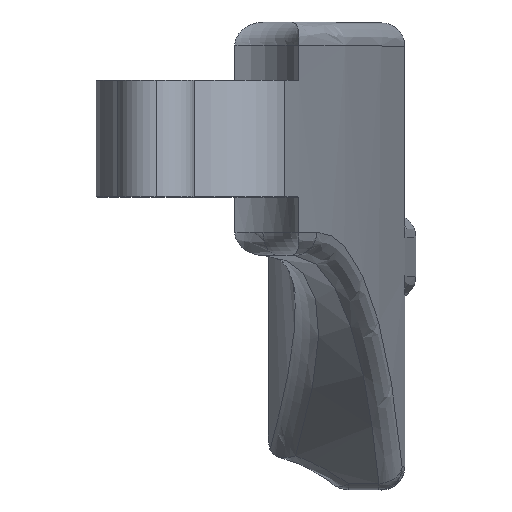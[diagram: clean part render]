
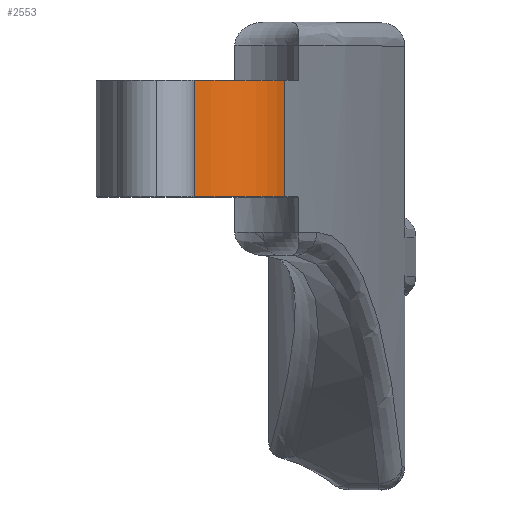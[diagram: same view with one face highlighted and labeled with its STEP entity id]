
A CAD part, top view. The second image highlights one B-rep face of the part: STEP entity #2553.
In plain terms, the highlighted cylindrical face has radius 12.6 mm (diameter 25.2 mm), a partial arc.
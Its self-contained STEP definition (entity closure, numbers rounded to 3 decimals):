
#46 = EDGE_LOOP ( 'NONE', ( #496, #1217, #1974, #1426 ) ) ;
#118 = EDGE_CURVE ( 'NONE', #2184, #1046, #1767, .T. ) ;
#164 = EDGE_CURVE ( 'NONE', #1065, #2184, #1087, .T. ) ;
#210 = LINE ( 'NONE', #1820, #586 ) ;
#295 = CIRCLE ( 'NONE', #1758, 12.6 ) ;
#458 = DIRECTION ( 'NONE',  ( 0., 1., 0. ) ) ;
#496 = ORIENTED_EDGE ( 'NONE', *, *, #118, .T. ) ;
#586 = VECTOR ( 'NONE', #1199, 1000. ) ;
#598 = FACE_OUTER_BOUND ( 'NONE', #46, .T. ) ;
#826 = CARTESIAN_POINT ( 'NONE',  ( 0., -60., 110. ) ) ;
#856 = DIRECTION ( 'NONE',  ( 0., -1., 0. ) ) ;
#911 = EDGE_CURVE ( 'NONE', #1065, #1109, #295, .T. ) ;
#976 = AXIS2_PLACEMENT_3D ( 'NONE', #1062, #856, #1874 ) ;
#1046 = VERTEX_POINT ( 'NONE', #1706 ) ;
#1062 = CARTESIAN_POINT ( 'NONE',  ( 0., -7.5, 110. ) ) ;
#1065 = VERTEX_POINT ( 'NONE', #1114 ) ;
#1067 = CARTESIAN_POINT ( 'NONE',  ( 0., -22.5, 110. ) ) ;
#1087 = LINE ( 'NONE', #2291, #1684 ) ;
#1109 = VERTEX_POINT ( 'NONE', #1577 ) ;
#1114 = CARTESIAN_POINT ( 'NONE',  ( 11.668, -22.5, 114.755 ) ) ;
#1199 = DIRECTION ( 'NONE',  ( 0., -1., 0. ) ) ;
#1217 = ORIENTED_EDGE ( 'NONE', *, *, #2532, .T. ) ;
#1294 = DIRECTION ( 'NONE',  ( 0., 0., -1. ) ) ;
#1399 = DIRECTION ( 'NONE',  ( 0., 0., -1. ) ) ;
#1426 = ORIENTED_EDGE ( 'NONE', *, *, #164, .T. ) ;
#1577 = CARTESIAN_POINT ( 'NONE',  ( 0.037, -22.5, 122.6 ) ) ;
#1581 = DIRECTION ( 'NONE',  ( 0., 1., 0. ) ) ;
#1684 = VECTOR ( 'NONE', #458, 1000. ) ;
#1706 = CARTESIAN_POINT ( 'NONE',  ( 0.037, -7.5, 122.6 ) ) ;
#1758 = AXIS2_PLACEMENT_3D ( 'NONE', #1067, #2287, #1294 ) ;
#1767 = CIRCLE ( 'NONE', #976, 12.6 ) ;
#1820 = CARTESIAN_POINT ( 'NONE',  ( 0.037, -15., 122.6 ) ) ;
#1874 = DIRECTION ( 'NONE',  ( 0., 0., -1. ) ) ;
#1974 = ORIENTED_EDGE ( 'NONE', *, *, #911, .F. ) ;
#2160 = CYLINDRICAL_SURFACE ( 'NONE', #2247, 12.6 ) ;
#2184 = VERTEX_POINT ( 'NONE', #2228 ) ;
#2228 = CARTESIAN_POINT ( 'NONE',  ( 11.668, -7.5, 114.755 ) ) ;
#2247 = AXIS2_PLACEMENT_3D ( 'NONE', #826, #1581, #1399 ) ;
#2287 = DIRECTION ( 'NONE',  ( 0., -1., 0. ) ) ;
#2291 = CARTESIAN_POINT ( 'NONE',  ( 11.668, -60., 114.755 ) ) ;
#2532 = EDGE_CURVE ( 'NONE', #1046, #1109, #210, .T. ) ;
#2553 = ADVANCED_FACE ( 'NONE', ( #598 ), #2160, .T. ) ;
